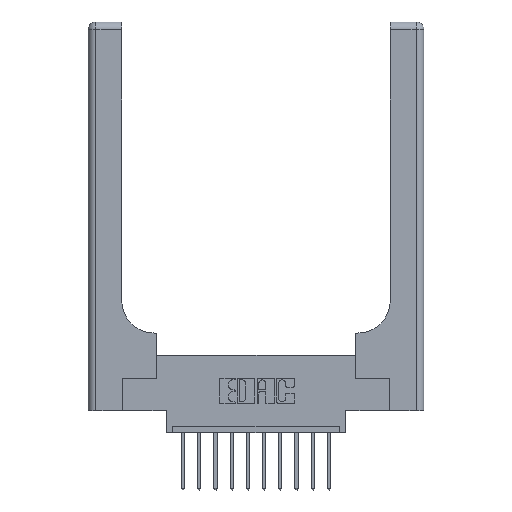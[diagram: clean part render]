
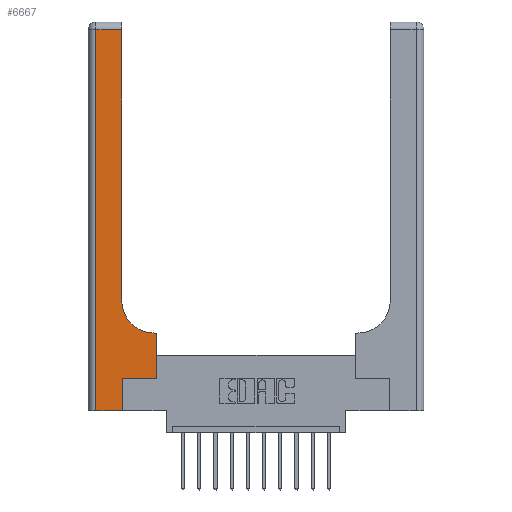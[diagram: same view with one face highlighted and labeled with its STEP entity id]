
A CAD part, top view. The second image highlights one B-rep face of the part: STEP entity #6667.
In plain terms, the highlighted planar face has unit normal (0, 0, 1).
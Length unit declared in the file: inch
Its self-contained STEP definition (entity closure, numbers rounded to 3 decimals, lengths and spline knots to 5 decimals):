
#342 = CARTESIAN_POINT ( 'NONE',  ( 0.265, 0.25, 0.37 ) ) ;
#381 = EDGE_CURVE ( 'NONE', #7052, #15680, #11811, .T. ) ;
#1041 = CARTESIAN_POINT ( 'NONE',  ( 0., 3., 0.37 ) ) ;
#1703 = AXIS2_PLACEMENT_3D ( 'NONE', #8530, #10938, #13596 ) ;
#1835 = CARTESIAN_POINT ( 'NONE',  ( 0., 2.94, 0.37 ) ) ;
#1962 = CIRCLE ( 'NONE', #1703, 0.25 ) ;
#2314 = LINE ( 'NONE', #7326, #6110 ) ;
#2609 = CARTESIAN_POINT ( 'NONE',  ( 0.528, 0.25, 0.37 ) ) ;
#2904 = VECTOR ( 'NONE', #12359, 39.37008 ) ;
#3023 = CARTESIAN_POINT ( 'NONE',  ( 0.51, 0.6, 0.37 ) ) ;
#3029 = ORIENTED_EDGE ( 'NONE', *, *, #381, .T. ) ;
#3205 = DIRECTION ( 'NONE',  ( -1., 0., 0. ) ) ;
#3393 = ORIENTED_EDGE ( 'NONE', *, *, #15900, .T. ) ;
#3564 = PLANE ( 'NONE',  #11598 ) ;
#3572 = VECTOR ( 'NONE', #3813, 39.37008 ) ;
#3589 = DIRECTION ( 'NONE',  ( -1., 0., 0. ) ) ;
#3813 = DIRECTION ( 'NONE',  ( 0., 1., 0. ) ) ;
#5107 = LINE ( 'NONE', #9929, #11373 ) ;
#5623 = EDGE_LOOP ( 'NONE', ( #12410, #3029, #5700, #3393, #9065, #12435, #8897, #11560, #5787 ) ) ;
#5700 = ORIENTED_EDGE ( 'NONE', *, *, #14696, .T. ) ;
#5787 = ORIENTED_EDGE ( 'NONE', *, *, #6730, .T. ) ;
#5889 = DIRECTION ( 'NONE',  ( -1., 0., 0. ) ) ;
#6110 = VECTOR ( 'NONE', #11138, 39.37008 ) ;
#6161 = CARTESIAN_POINT ( 'NONE',  ( 0.26, 0.6, 0.37 ) ) ;
#6667 = ADVANCED_FACE ( 'NONE', ( #11020 ), #3564, .F. ) ;
#6730 = EDGE_CURVE ( 'NONE', #14337, #7951, #1962, .T. ) ;
#6782 = VECTOR ( 'NONE', #8730, 39.37008 ) ;
#6888 = CARTESIAN_POINT ( 'NONE',  ( 0.528, 0.25, 0.37 ) ) ;
#7052 = VERTEX_POINT ( 'NONE', #12084 ) ;
#7326 = CARTESIAN_POINT ( 'NONE',  ( 0., 0., 0.37 ) ) ;
#7581 = LINE ( 'NONE', #10067, #6782 ) ;
#7951 = VERTEX_POINT ( 'NONE', #8078 ) ;
#8078 = CARTESIAN_POINT ( 'NONE',  ( 0.26, 0.85, 0.37 ) ) ;
#8103 = DIRECTION ( 'NONE',  ( 0., -1., 0. ) ) ;
#8462 = CARTESIAN_POINT ( 'NONE',  ( 0.265, 0., 0.37 ) ) ;
#8530 = CARTESIAN_POINT ( 'NONE',  ( 0.51, 0.85, 0.37 ) ) ;
#8552 = LINE ( 'NONE', #6161, #8973 ) ;
#8631 = EDGE_CURVE ( 'NONE', #9706, #14578, #10103, .T. ) ;
#8730 = DIRECTION ( 'NONE',  ( 0., 1., 0. ) ) ;
#8777 = LINE ( 'NONE', #14015, #12097 ) ;
#8835 = EDGE_CURVE ( 'NONE', #12975, #16026, #7581, .T. ) ;
#8897 = ORIENTED_EDGE ( 'NONE', *, *, #8631, .T. ) ;
#8973 = VECTOR ( 'NONE', #3589, 39.37008 ) ;
#9065 = ORIENTED_EDGE ( 'NONE', *, *, #8835, .T. ) ;
#9324 = EDGE_CURVE ( 'NONE', #14578, #14337, #8552, .T. ) ;
#9573 = VECTOR ( 'NONE', #3205, 39.37008 ) ;
#9706 = VERTEX_POINT ( 'NONE', #6888 ) ;
#9838 = CARTESIAN_POINT ( 'NONE',  ( 0.06, 0., 0.37 ) ) ;
#9929 = CARTESIAN_POINT ( 'NONE',  ( 0.06, 3., 0.37 ) ) ;
#10067 = CARTESIAN_POINT ( 'NONE',  ( 0.265, 0., 0.37 ) ) ;
#10103 = LINE ( 'NONE', #2609, #3572 ) ;
#10938 = DIRECTION ( 'NONE',  ( 0., 0., -1. ) ) ;
#11020 = FACE_OUTER_BOUND ( 'NONE', #5623, .T. ) ;
#11138 = DIRECTION ( 'NONE',  ( 1., 0., 0. ) ) ;
#11373 = VECTOR ( 'NONE', #8103, 39.37008 ) ;
#11560 = ORIENTED_EDGE ( 'NONE', *, *, #9324, .T. ) ;
#11598 = AXIS2_PLACEMENT_3D ( 'NONE', #1041, #12267, #5889 ) ;
#11811 = LINE ( 'NONE', #1835, #9573 ) ;
#11882 = EDGE_CURVE ( 'NONE', #16026, #9706, #8777, .T. ) ;
#12084 = CARTESIAN_POINT ( 'NONE',  ( 0.26, 2.94, 0.37 ) ) ;
#12097 = VECTOR ( 'NONE', #12524, 39.37008 ) ;
#12267 = DIRECTION ( 'NONE',  ( 0., 0., -1. ) ) ;
#12359 = DIRECTION ( 'NONE',  ( 0., 1., 0. ) ) ;
#12410 = ORIENTED_EDGE ( 'NONE', *, *, #12943, .T. ) ;
#12435 = ORIENTED_EDGE ( 'NONE', *, *, #11882, .T. ) ;
#12524 = DIRECTION ( 'NONE',  ( 1., 0., 0. ) ) ;
#12669 = CARTESIAN_POINT ( 'NONE',  ( 0.528, 0.6, 0.37 ) ) ;
#12943 = EDGE_CURVE ( 'NONE', #7951, #7052, #14681, .T. ) ;
#12975 = VERTEX_POINT ( 'NONE', #8462 ) ;
#13337 = VERTEX_POINT ( 'NONE', #9838 ) ;
#13596 = DIRECTION ( 'NONE',  ( 1., 0., 0. ) ) ;
#14015 = CARTESIAN_POINT ( 'NONE',  ( 0.265, 0.25, 0.37 ) ) ;
#14337 = VERTEX_POINT ( 'NONE', #3023 ) ;
#14578 = VERTEX_POINT ( 'NONE', #12669 ) ;
#14681 = LINE ( 'NONE', #15959, #2904 ) ;
#14696 = EDGE_CURVE ( 'NONE', #15680, #13337, #5107, .T. ) ;
#15316 = CARTESIAN_POINT ( 'NONE',  ( 0.06, 2.94, 0.37 ) ) ;
#15680 = VERTEX_POINT ( 'NONE', #15316 ) ;
#15900 = EDGE_CURVE ( 'NONE', #13337, #12975, #2314, .T. ) ;
#15959 = CARTESIAN_POINT ( 'NONE',  ( 0.26, 3., 0.37 ) ) ;
#16026 = VERTEX_POINT ( 'NONE', #342 ) ;
